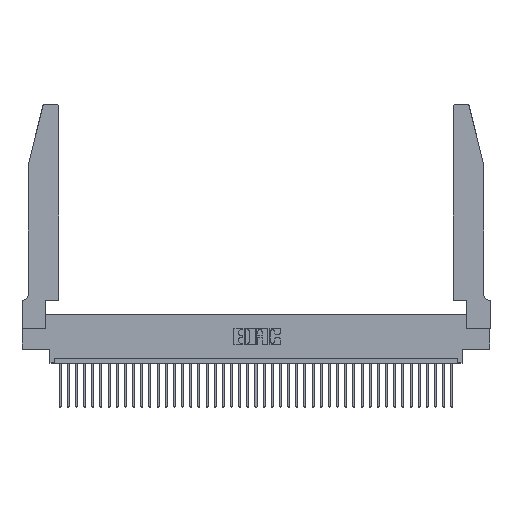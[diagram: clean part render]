
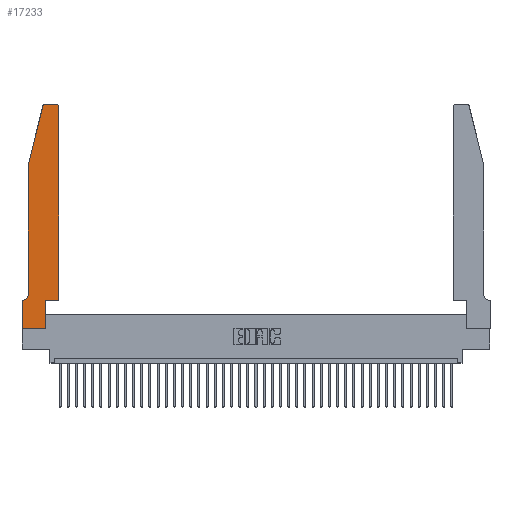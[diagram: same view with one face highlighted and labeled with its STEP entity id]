
A CAD part, top view. The second image highlights one B-rep face of the part: STEP entity #17233.
In plain terms, the highlighted planar face has unit normal (0, 0, 1).
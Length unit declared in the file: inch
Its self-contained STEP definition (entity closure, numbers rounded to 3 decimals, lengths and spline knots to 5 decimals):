
#493 = VECTOR ( 'NONE', #23178, 39.37008 ) ;
#701 = CARTESIAN_POINT ( 'NONE',  ( 0.4505, 0.35, 0.37 ) ) ;
#963 = VECTOR ( 'NONE', #27354, 39.37008 ) ;
#1228 = DIRECTION ( 'NONE',  ( 0., 0., 1. ) ) ;
#1349 = VECTOR ( 'NONE', #14798, 39.37008 ) ;
#1845 = LINE ( 'NONE', #11305, #1349 ) ;
#1994 = LINE ( 'NONE', #23009, #6858 ) ;
#2145 = CARTESIAN_POINT ( 'NONE',  ( 0., 0., 0.37 ) ) ;
#2418 = ORIENTED_EDGE ( 'NONE', *, *, #14465, .T. ) ;
#2974 = CARTESIAN_POINT ( 'NONE',  ( 0.0755, 2., 0.37 ) ) ;
#3225 = VERTEX_POINT ( 'NONE', #14327 ) ;
#3707 = VERTEX_POINT ( 'NONE', #25308 ) ;
#4395 = CARTESIAN_POINT ( 'NONE',  ( 0.0755, 2., 0.37 ) ) ;
#4690 = CARTESIAN_POINT ( 'NONE',  ( 0.2605, 2.75, 0.37 ) ) ;
#4877 = CARTESIAN_POINT ( 'NONE',  ( 0.4505, 2.72, 0.37 ) ) ;
#6381 = ORIENTED_EDGE ( 'NONE', *, *, #21176, .T. ) ;
#6684 = CARTESIAN_POINT ( 'NONE',  ( 0.0055, 0.42, 0.37 ) ) ;
#6835 = LINE ( 'NONE', #4690, #38423 ) ;
#6858 = VECTOR ( 'NONE', #16528, 39.37008 ) ;
#6885 = EDGE_LOOP ( 'NONE', ( #28445, #9362, #2418, #22468, #29657, #24299, #24809, #6381, #9706, #35395, #19688, #22815 ) ) ;
#7102 = FACE_OUTER_BOUND ( 'NONE', #6885, .T. ) ;
#7870 = VERTEX_POINT ( 'NONE', #17372 ) ;
#7897 = CARTESIAN_POINT ( 'NONE',  ( 0.4205, 2.72, 0.37 ) ) ;
#8152 = CARTESIAN_POINT ( 'NONE',  ( 0.2865, 0.35, 0.37 ) ) ;
#8320 = DIRECTION ( 'NONE',  ( -1., 0., 0. ) ) ;
#8801 = CIRCLE ( 'NONE', #19798, 0.03 ) ;
#9362 = ORIENTED_EDGE ( 'NONE', *, *, #31826, .T. ) ;
#9598 = CARTESIAN_POINT ( 'NONE',  ( 0.284, 2.72, 0.37 ) ) ;
#9706 = ORIENTED_EDGE ( 'NONE', *, *, #9886, .T. ) ;
#9886 = EDGE_CURVE ( 'NONE', #7870, #3707, #27641, .T. ) ;
#9959 = LINE ( 'NONE', #2145, #30847 ) ;
#10215 = DIRECTION ( 'NONE',  ( 1., 0., 0. ) ) ;
#10635 = CARTESIAN_POINT ( 'NONE',  ( 0., 0.35, 0.37 ) ) ;
#11137 = EDGE_CURVE ( 'NONE', #14829, #25756, #9959, .T. ) ;
#11305 = CARTESIAN_POINT ( 'NONE',  ( 0.0755, 2., 0.37 ) ) ;
#12293 = CARTESIAN_POINT ( 'NONE',  ( 0.25487, 2.72718, 0.37 ) ) ;
#12365 = AXIS2_PLACEMENT_3D ( 'NONE', #22678, #19807, #26098 ) ;
#12888 = EDGE_CURVE ( 'NONE', #23807, #39118, #31152, .T. ) ;
#13809 = CARTESIAN_POINT ( 'NONE',  ( 0.4505, 0.35, 0.37 ) ) ;
#13829 = VECTOR ( 'NONE', #10215, 39.37008 ) ;
#13897 = VECTOR ( 'NONE', #8320, 39.37008 ) ;
#14327 = CARTESIAN_POINT ( 'NONE',  ( 0.0055, 0.35, 0.37 ) ) ;
#14465 = EDGE_CURVE ( 'NONE', #26158, #33897, #40864, .T. ) ;
#14798 = DIRECTION ( 'NONE',  ( 0., -1., 0. ) ) ;
#14829 = VERTEX_POINT ( 'NONE', #10635 ) ;
#14887 = LINE ( 'NONE', #19256, #13829 ) ;
#15796 = CARTESIAN_POINT ( 'NONE',  ( 0.284, 2.75, 0.37 ) ) ;
#16528 = DIRECTION ( 'NONE',  ( 1., 0., 0. ) ) ;
#16667 = DIRECTION ( 'NONE',  ( -0.239, -0.971, 0. ) ) ;
#16943 = VERTEX_POINT ( 'NONE', #15796 ) ;
#17184 = DIRECTION ( 'NONE',  ( -1., 0., 0. ) ) ;
#17233 = ADVANCED_FACE ( 'NONE', ( #7102 ), #25806, .T. ) ;
#17372 = CARTESIAN_POINT ( 'NONE',  ( 0.2865, 0., 0.37 ) ) ;
#17557 = DIRECTION ( 'NONE',  ( -1., 0., 0. ) ) ;
#17763 = AXIS2_PLACEMENT_3D ( 'NONE', #7897, #26373, #29855 ) ;
#19256 = CARTESIAN_POINT ( 'NONE',  ( 0., 0., 0.37 ) ) ;
#19688 = ORIENTED_EDGE ( 'NONE', *, *, #12888, .T. ) ;
#19798 = AXIS2_PLACEMENT_3D ( 'NONE', #9598, #1228, #23287 ) ;
#19807 = DIRECTION ( 'NONE',  ( 0., 0., 1. ) ) ;
#19847 = EDGE_CURVE ( 'NONE', #3225, #14829, #22273, .T. ) ;
#19977 = EDGE_CURVE ( 'NONE', #22077, #3225, #25254, .T. ) ;
#21086 = CARTESIAN_POINT ( 'NONE',  ( 0.0755, 0.35, 0.37 ) ) ;
#21176 = EDGE_CURVE ( 'NONE', #25756, #7870, #14887, .T. ) ;
#21254 = CIRCLE ( 'NONE', #17763, 0.03 ) ;
#21704 = EDGE_CURVE ( 'NONE', #39118, #33869, #21254, .T. ) ;
#21828 = EDGE_CURVE ( 'NONE', #33869, #16943, #6835, .T. ) ;
#22077 = VERTEX_POINT ( 'NONE', #29404 ) ;
#22273 = LINE ( 'NONE', #21086, #13897 ) ;
#22468 = ORIENTED_EDGE ( 'NONE', *, *, #25033, .T. ) ;
#22678 = CARTESIAN_POINT ( 'NONE',  ( 0., 0.35, 0.37 ) ) ;
#22815 = ORIENTED_EDGE ( 'NONE', *, *, #21704, .T. ) ;
#23009 = CARTESIAN_POINT ( 'NONE',  ( 0.4505, 0.35, 0.37 ) ) ;
#23178 = DIRECTION ( 'NONE',  ( 0., 1., 0. ) ) ;
#23287 = DIRECTION ( 'NONE',  ( 1., 0., 0. ) ) ;
#23807 = VERTEX_POINT ( 'NONE', #701 ) ;
#24194 = DIRECTION ( 'NONE',  ( 0., -1., 0. ) ) ;
#24299 = ORIENTED_EDGE ( 'NONE', *, *, #19847, .T. ) ;
#24809 = ORIENTED_EDGE ( 'NONE', *, *, #11137, .T. ) ;
#25033 = EDGE_CURVE ( 'NONE', #33897, #22077, #1845, .T. ) ;
#25176 = CARTESIAN_POINT ( 'NONE',  ( 0., 0., 0.37 ) ) ;
#25254 = CIRCLE ( 'NONE', #30716, 0.07 ) ;
#25308 = CARTESIAN_POINT ( 'NONE',  ( 0.2865, 0.35, 0.37 ) ) ;
#25756 = VERTEX_POINT ( 'NONE', #25176 ) ;
#25806 = PLANE ( 'NONE',  #12365 ) ;
#26098 = DIRECTION ( 'NONE',  ( 1., 0., 0. ) ) ;
#26158 = VERTEX_POINT ( 'NONE', #12293 ) ;
#26373 = DIRECTION ( 'NONE',  ( 0., 0., 1. ) ) ;
#27354 = DIRECTION ( 'NONE',  ( 0., 1., 0. ) ) ;
#27641 = LINE ( 'NONE', #8152, #963 ) ;
#27731 = EDGE_CURVE ( 'NONE', #3707, #23807, #1994, .T. ) ;
#28445 = ORIENTED_EDGE ( 'NONE', *, *, #21828, .T. ) ;
#29404 = CARTESIAN_POINT ( 'NONE',  ( 0.0755, 0.42, 0.37 ) ) ;
#29657 = ORIENTED_EDGE ( 'NONE', *, *, #19977, .T. ) ;
#29855 = DIRECTION ( 'NONE',  ( 1., 0., 0. ) ) ;
#30716 = AXIS2_PLACEMENT_3D ( 'NONE', #6684, #32051, #17184 ) ;
#30847 = VECTOR ( 'NONE', #24194, 39.37008 ) ;
#31152 = LINE ( 'NONE', #13809, #493 ) ;
#31167 = CARTESIAN_POINT ( 'NONE',  ( 0.4205, 2.75, 0.37 ) ) ;
#31826 = EDGE_CURVE ( 'NONE', #16943, #26158, #8801, .T. ) ;
#32051 = DIRECTION ( 'NONE',  ( 0., 0., -1. ) ) ;
#33869 = VERTEX_POINT ( 'NONE', #31167 ) ;
#33897 = VERTEX_POINT ( 'NONE', #2974 ) ;
#34919 = VECTOR ( 'NONE', #16667, 39.37008 ) ;
#35395 = ORIENTED_EDGE ( 'NONE', *, *, #27731, .T. ) ;
#38423 = VECTOR ( 'NONE', #17557, 39.37008 ) ;
#39118 = VERTEX_POINT ( 'NONE', #4877 ) ;
#40864 = LINE ( 'NONE', #4395, #34919 ) ;
